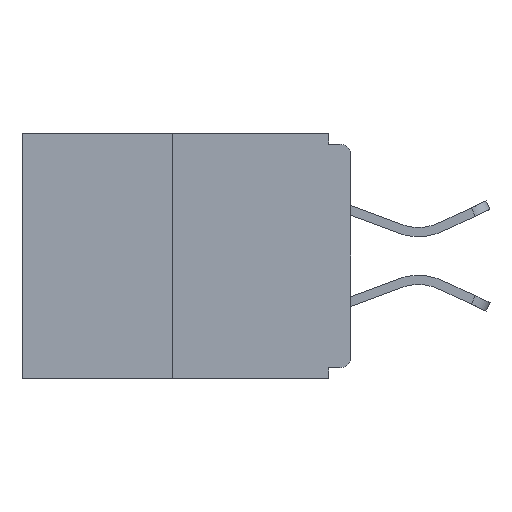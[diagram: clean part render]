
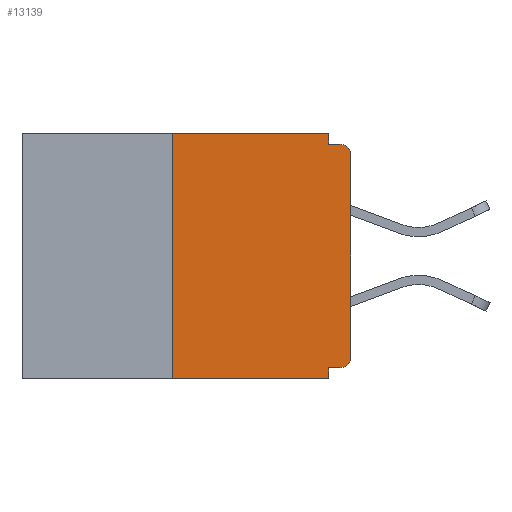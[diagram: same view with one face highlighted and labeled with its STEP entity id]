
A CAD part, left-side view. The second image highlights one B-rep face of the part: STEP entity #13139.
In plain terms, the highlighted planar face has unit normal (-1, 0, 0).
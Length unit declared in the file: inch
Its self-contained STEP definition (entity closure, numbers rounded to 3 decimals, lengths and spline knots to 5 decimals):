
#56 = CARTESIAN_POINT ( 'NONE',  ( 0., 0.031, -0.343 ) ) ;
#157 = DIRECTION ( 'NONE',  ( 0., 0., -1. ) ) ;
#689 = CARTESIAN_POINT ( 'NONE',  ( 0., 0.25, -0.343 ) ) ;
#795 = CARTESIAN_POINT ( 'NONE',  ( 0., 0.031, -0.015 ) ) ;
#1415 = VERTEX_POINT ( 'NONE', #3118 ) ;
#1549 = VERTEX_POINT ( 'NONE', #5395 ) ;
#1646 = EDGE_CURVE ( 'NONE', #2146, #11257, #11139, .T. ) ;
#1657 = VERTEX_POINT ( 'NONE', #11709 ) ;
#2047 = CARTESIAN_POINT ( 'NONE',  ( 0., 0.015, -0.015 ) ) ;
#2111 = VECTOR ( 'NONE', #10193, 39.37008 ) ;
#2146 = VERTEX_POINT ( 'NONE', #17017 ) ;
#2396 = CARTESIAN_POINT ( 'NONE',  ( 0., 0.015, -0.313 ) ) ;
#2615 = EDGE_LOOP ( 'NONE', ( #4745, #3262, #16425, #3764, #15254, #12735, #5660, #18037, #8556, #14996 ) ) ;
#2626 = EDGE_CURVE ( 'NONE', #1657, #3688, #2653, .T. ) ;
#2653 = CIRCLE ( 'NONE', #17711, 0.015 ) ;
#2666 = LINE ( 'NONE', #2856, #14328 ) ;
#2856 = CARTESIAN_POINT ( 'NONE',  ( 0., 0.46, -0.343 ) ) ;
#3118 = CARTESIAN_POINT ( 'NONE',  ( 0., 0.25, 0. ) ) ;
#3262 = ORIENTED_EDGE ( 'NONE', *, *, #13876, .F. ) ;
#3588 = VECTOR ( 'NONE', #4433, 39.37008 ) ;
#3639 = DIRECTION ( 'NONE',  ( 0., 1., 0. ) ) ;
#3688 = VERTEX_POINT ( 'NONE', #2047 ) ;
#3764 = ORIENTED_EDGE ( 'NONE', *, *, #12674, .F. ) ;
#4089 = DIRECTION ( 'NONE',  ( 0., 0., -1. ) ) ;
#4244 = DIRECTION ( 'NONE',  ( 0., -1., 0. ) ) ;
#4433 = DIRECTION ( 'NONE',  ( 0., -1., 0. ) ) ;
#4745 = ORIENTED_EDGE ( 'NONE', *, *, #17279, .F. ) ;
#4812 = VERTEX_POINT ( 'NONE', #15926 ) ;
#5077 = AXIS2_PLACEMENT_3D ( 'NONE', #15958, #9055, #14678 ) ;
#5395 = CARTESIAN_POINT ( 'NONE',  ( 0., 0.031, -0.343 ) ) ;
#5660 = ORIENTED_EDGE ( 'NONE', *, *, #6148, .T. ) ;
#6148 = EDGE_CURVE ( 'NONE', #9744, #1657, #10128, .T. ) ;
#7455 = VECTOR ( 'NONE', #157, 39.37008 ) ;
#7649 = FACE_OUTER_BOUND ( 'NONE', #2615, .T. ) ;
#8556 = ORIENTED_EDGE ( 'NONE', *, *, #17284, .F. ) ;
#8657 = CARTESIAN_POINT ( 'NONE',  ( 0., 0., 0. ) ) ;
#8793 = CARTESIAN_POINT ( 'NONE',  ( 0., 0.015, -0.03 ) ) ;
#9055 = DIRECTION ( 'NONE',  ( 1., 0., 0. ) ) ;
#9380 = EDGE_CURVE ( 'NONE', #11721, #1549, #2666, .T. ) ;
#9483 = CIRCLE ( 'NONE', #11859, 0.015 ) ;
#9507 = CARTESIAN_POINT ( 'NONE',  ( 0., 0., -0.313 ) ) ;
#9633 = CARTESIAN_POINT ( 'NONE',  ( 0., 0.25, 0. ) ) ;
#9744 = VERTEX_POINT ( 'NONE', #9507 ) ;
#10000 = CARTESIAN_POINT ( 'NONE',  ( 0., 0., -0.015 ) ) ;
#10117 = VECTOR ( 'NONE', #4089, 39.37008 ) ;
#10128 = LINE ( 'NONE', #8657, #15037 ) ;
#10193 = DIRECTION ( 'NONE',  ( 0., -1., 0. ) ) ;
#10526 = CARTESIAN_POINT ( 'NONE',  ( 0., 0.46, 0. ) ) ;
#11139 = LINE ( 'NONE', #16764, #10117 ) ;
#11257 = VERTEX_POINT ( 'NONE', #795 ) ;
#11319 = VECTOR ( 'NONE', #15260, 39.37008 ) ;
#11466 = LINE ( 'NONE', #11658, #12467 ) ;
#11470 = DIRECTION ( 'NONE',  ( -1., 0., 0. ) ) ;
#11642 = PLANE ( 'NONE',  #5077 ) ;
#11658 = CARTESIAN_POINT ( 'NONE',  ( 0., 0., -0.328 ) ) ;
#11674 = CARTESIAN_POINT ( 'NONE',  ( 0., 0.031, -0.328 ) ) ;
#11709 = CARTESIAN_POINT ( 'NONE',  ( 0., 0., -0.03 ) ) ;
#11721 = VERTEX_POINT ( 'NONE', #689 ) ;
#11859 = AXIS2_PLACEMENT_3D ( 'NONE', #2396, #16255, #15056 ) ;
#12467 = VECTOR ( 'NONE', #3639, 39.37008 ) ;
#12674 = EDGE_CURVE ( 'NONE', #14152, #1549, #16878, .T. ) ;
#12735 = ORIENTED_EDGE ( 'NONE', *, *, #16605, .T. ) ;
#13139 = ADVANCED_FACE ( 'NONE', ( #7649 ), #11642, .F. ) ;
#13876 = EDGE_CURVE ( 'NONE', #11721, #1415, #17849, .T. ) ;
#14152 = VERTEX_POINT ( 'NONE', #11674 ) ;
#14328 = VECTOR ( 'NONE', #4244, 39.37008 ) ;
#14678 = DIRECTION ( 'NONE',  ( 0., 0., -1. ) ) ;
#14996 = ORIENTED_EDGE ( 'NONE', *, *, #1646, .F. ) ;
#15037 = VECTOR ( 'NONE', #17128, 39.37008 ) ;
#15056 = DIRECTION ( 'NONE',  ( 0., 0., -1. ) ) ;
#15254 = ORIENTED_EDGE ( 'NONE', *, *, #17613, .F. ) ;
#15260 = DIRECTION ( 'NONE',  ( 0., 0., 1. ) ) ;
#15820 = LINE ( 'NONE', #10000, #3588 ) ;
#15926 = CARTESIAN_POINT ( 'NONE',  ( 0., 0.015, -0.328 ) ) ;
#15958 = CARTESIAN_POINT ( 'NONE',  ( 0., 0.46, 0. ) ) ;
#16255 = DIRECTION ( 'NONE',  ( -1., 0., 0. ) ) ;
#16425 = ORIENTED_EDGE ( 'NONE', *, *, #9380, .T. ) ;
#16605 = EDGE_CURVE ( 'NONE', #4812, #9744, #9483, .T. ) ;
#16764 = CARTESIAN_POINT ( 'NONE',  ( 0., 0.031, 0. ) ) ;
#16878 = LINE ( 'NONE', #56, #7455 ) ;
#17017 = CARTESIAN_POINT ( 'NONE',  ( 0., 0.031, 0. ) ) ;
#17082 = DIRECTION ( 'NONE',  ( 0., 0., -1. ) ) ;
#17128 = DIRECTION ( 'NONE',  ( 0., 0., 1. ) ) ;
#17191 = LINE ( 'NONE', #10526, #2111 ) ;
#17279 = EDGE_CURVE ( 'NONE', #1415, #2146, #17191, .T. ) ;
#17284 = EDGE_CURVE ( 'NONE', #11257, #3688, #15820, .T. ) ;
#17613 = EDGE_CURVE ( 'NONE', #4812, #14152, #11466, .T. ) ;
#17711 = AXIS2_PLACEMENT_3D ( 'NONE', #8793, #11470, #17082 ) ;
#17849 = LINE ( 'NONE', #9633, #11319 ) ;
#18037 = ORIENTED_EDGE ( 'NONE', *, *, #2626, .T. ) ;
